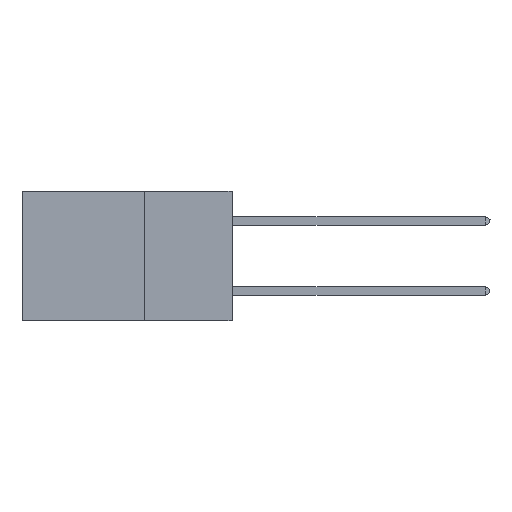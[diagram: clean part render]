
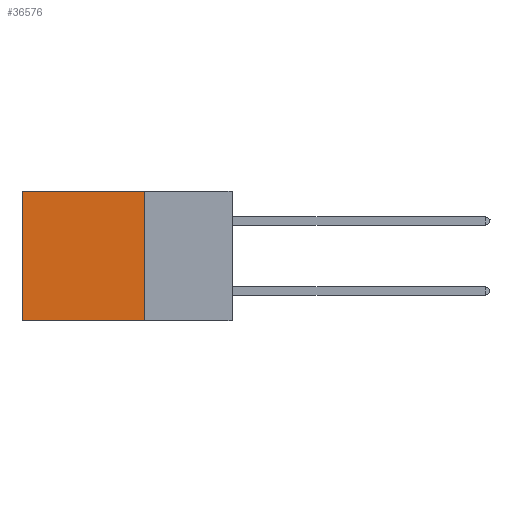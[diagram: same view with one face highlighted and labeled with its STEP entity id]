
A CAD part, left-side view. The second image highlights one B-rep face of the part: STEP entity #36576.
In plain terms, the highlighted planar face has unit normal (-1, 0, 0).
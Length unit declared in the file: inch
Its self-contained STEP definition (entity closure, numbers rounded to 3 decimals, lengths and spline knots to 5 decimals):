
#231 = CARTESIAN_POINT ( 'NONE',  ( 0.2875, 0.6, -0.37 ) ) ;
#2520 = EDGE_CURVE ( 'NONE', #45002, #23560, #28018, .T. ) ;
#3772 = DIRECTION ( 'NONE',  ( 0., 1., 0. ) ) ;
#3865 = CARTESIAN_POINT ( 'NONE',  ( 0.2875, 0.6, 0. ) ) ;
#5224 = ORIENTED_EDGE ( 'NONE', *, *, #36301, .F. ) ;
#6232 = CARTESIAN_POINT ( 'NONE',  ( 0.2875, 0.6, 0. ) ) ;
#6657 = VERTEX_POINT ( 'NONE', #28381 ) ;
#8569 = EDGE_CURVE ( 'NONE', #23287, #45002, #33870, .T. ) ;
#9531 = CARTESIAN_POINT ( 'NONE',  ( 0.2875, 0.25, 0. ) ) ;
#10486 = CARTESIAN_POINT ( 'NONE',  ( 0.2875, 0.25, -0.37 ) ) ;
#12292 = VECTOR ( 'NONE', #23662, 39.37008 ) ;
#15362 = ORIENTED_EDGE ( 'NONE', *, *, #8569, .T. ) ;
#16424 = VECTOR ( 'NONE', #3772, 39.37008 ) ;
#17009 = EDGE_LOOP ( 'NONE', ( #23407, #21874, #5224, #15362 ) ) ;
#17217 = LINE ( 'NONE', #10486, #16424 ) ;
#18514 = DIRECTION ( 'NONE',  ( 0., 0., -1. ) ) ;
#20724 = FACE_OUTER_BOUND ( 'NONE', #17009, .T. ) ;
#21874 = ORIENTED_EDGE ( 'NONE', *, *, #24367, .F. ) ;
#23287 = VERTEX_POINT ( 'NONE', #43369 ) ;
#23407 = ORIENTED_EDGE ( 'NONE', *, *, #2520, .T. ) ;
#23560 = VERTEX_POINT ( 'NONE', #231 ) ;
#23662 = DIRECTION ( 'NONE',  ( 0., 1., 0. ) ) ;
#24367 = EDGE_CURVE ( 'NONE', #6657, #23560, #17217, .T. ) ;
#25248 = DIRECTION ( 'NONE',  ( 0., 0., -1. ) ) ;
#27249 = PLANE ( 'NONE',  #36953 ) ;
#28018 = LINE ( 'NONE', #3865, #28327 ) ;
#28327 = VECTOR ( 'NONE', #25248, 39.37008 ) ;
#28381 = CARTESIAN_POINT ( 'NONE',  ( 0.2875, 0.25, -0.37 ) ) ;
#33249 = VECTOR ( 'NONE', #18514, 39.37008 ) ;
#33870 = LINE ( 'NONE', #9531, #12292 ) ;
#36301 = EDGE_CURVE ( 'NONE', #23287, #6657, #37456, .T. ) ;
#36576 = ADVANCED_FACE ( 'NONE', ( #20724 ), #27249, .F. ) ;
#36953 = AXIS2_PLACEMENT_3D ( 'NONE', #41830, #45537, #42052 ) ;
#37456 = LINE ( 'NONE', #40940, #33249 ) ;
#40940 = CARTESIAN_POINT ( 'NONE',  ( 0.2875, 0.25, 0. ) ) ;
#41830 = CARTESIAN_POINT ( 'NONE',  ( 0.2875, 0.25, 0. ) ) ;
#42052 = DIRECTION ( 'NONE',  ( 0., 0., -1. ) ) ;
#43369 = CARTESIAN_POINT ( 'NONE',  ( 0.2875, 0.25, 0. ) ) ;
#45002 = VERTEX_POINT ( 'NONE', #6232 ) ;
#45537 = DIRECTION ( 'NONE',  ( 1., 0., 0. ) ) ;
